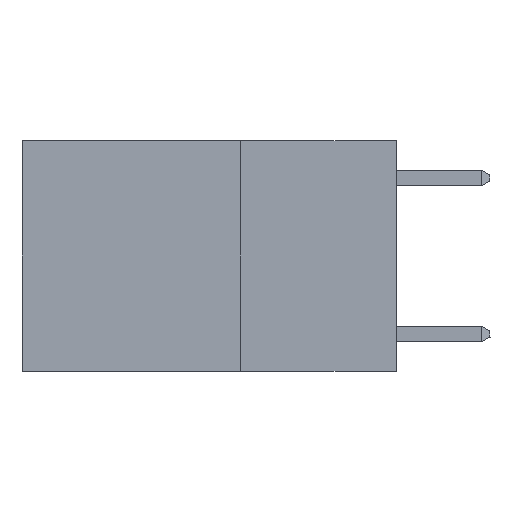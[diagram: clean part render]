
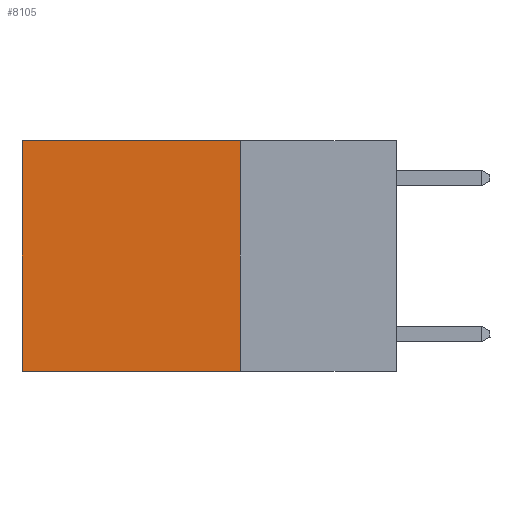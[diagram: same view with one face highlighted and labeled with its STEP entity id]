
A CAD part, left-side view. The second image highlights one B-rep face of the part: STEP entity #8105.
In plain terms, the highlighted planar face has unit normal (-1, 0, 0).
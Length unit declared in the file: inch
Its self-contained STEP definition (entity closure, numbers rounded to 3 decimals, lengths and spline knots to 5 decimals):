
#36 = PLANE ( 'NONE',  #9748 ) ;
#180 = DIRECTION ( 'NONE',  ( 0., 1., 0. ) ) ;
#808 = VERTEX_POINT ( 'NONE', #8230 ) ;
#1118 = VERTEX_POINT ( 'NONE', #2197 ) ;
#1128 = CARTESIAN_POINT ( 'NONE',  ( 0.2625, 0.25, 0. ) ) ;
#1860 = EDGE_CURVE ( 'NONE', #3623, #1118, #6728, .T. ) ;
#2011 = LINE ( 'NONE', #1128, #12347 ) ;
#2063 = DIRECTION ( 'NONE',  ( 1., 0., 0. ) ) ;
#2197 = CARTESIAN_POINT ( 'NONE',  ( 0.2625, 0.6, 0. ) ) ;
#2859 = EDGE_CURVE ( 'NONE', #808, #10262, #6228, .T. ) ;
#2927 = CARTESIAN_POINT ( 'NONE',  ( 0.2625, 0.25, 0. ) ) ;
#3082 = DIRECTION ( 'NONE',  ( 0., 0., -1. ) ) ;
#3470 = CARTESIAN_POINT ( 'NONE',  ( 0.2625, 0.6, -0.37 ) ) ;
#3623 = VERTEX_POINT ( 'NONE', #5867 ) ;
#4106 = VECTOR ( 'NONE', #5651, 39.37008 ) ;
#4156 = ORIENTED_EDGE ( 'NONE', *, *, #9452, .F. ) ;
#4625 = CARTESIAN_POINT ( 'NONE',  ( 0.2625, 0.6, 0. ) ) ;
#4793 = EDGE_LOOP ( 'NONE', ( #11476, #9191, #4156, #9495 ) ) ;
#4794 = FACE_OUTER_BOUND ( 'NONE', #4793, .T. ) ;
#5122 = DIRECTION ( 'NONE',  ( 0., 1., 0. ) ) ;
#5651 = DIRECTION ( 'NONE',  ( 0., 0., -1. ) ) ;
#5867 = CARTESIAN_POINT ( 'NONE',  ( 0.2625, 0.25, 0. ) ) ;
#6228 = LINE ( 'NONE', #12741, #11188 ) ;
#6728 = LINE ( 'NONE', #2927, #8460 ) ;
#7157 = CARTESIAN_POINT ( 'NONE',  ( 0.2625, 0.25, 0. ) ) ;
#8105 = ADVANCED_FACE ( 'NONE', ( #4794 ), #36, .F. ) ;
#8230 = CARTESIAN_POINT ( 'NONE',  ( 0.2625, 0.25, -0.37 ) ) ;
#8460 = VECTOR ( 'NONE', #5122, 39.37008 ) ;
#9180 = DIRECTION ( 'NONE',  ( 0., 0., -1. ) ) ;
#9191 = ORIENTED_EDGE ( 'NONE', *, *, #2859, .F. ) ;
#9452 = EDGE_CURVE ( 'NONE', #3623, #808, #2011, .T. ) ;
#9495 = ORIENTED_EDGE ( 'NONE', *, *, #1860, .T. ) ;
#9743 = LINE ( 'NONE', #4625, #4106 ) ;
#9748 = AXIS2_PLACEMENT_3D ( 'NONE', #7157, #2063, #9180 ) ;
#10262 = VERTEX_POINT ( 'NONE', #3470 ) ;
#11149 = EDGE_CURVE ( 'NONE', #1118, #10262, #9743, .T. ) ;
#11188 = VECTOR ( 'NONE', #180, 39.37008 ) ;
#11476 = ORIENTED_EDGE ( 'NONE', *, *, #11149, .T. ) ;
#12347 = VECTOR ( 'NONE', #3082, 39.37008 ) ;
#12741 = CARTESIAN_POINT ( 'NONE',  ( 0.2625, 0.25, -0.37 ) ) ;
